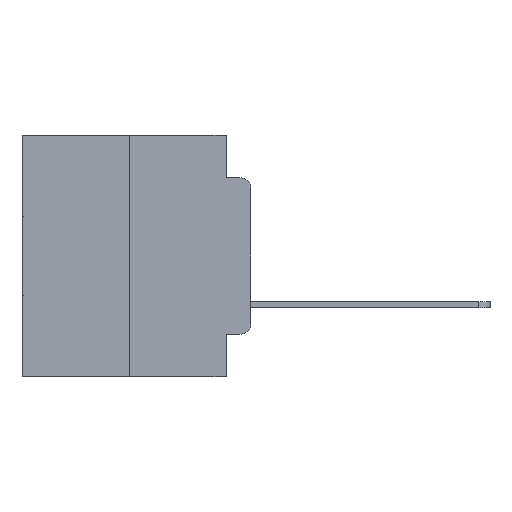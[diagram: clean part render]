
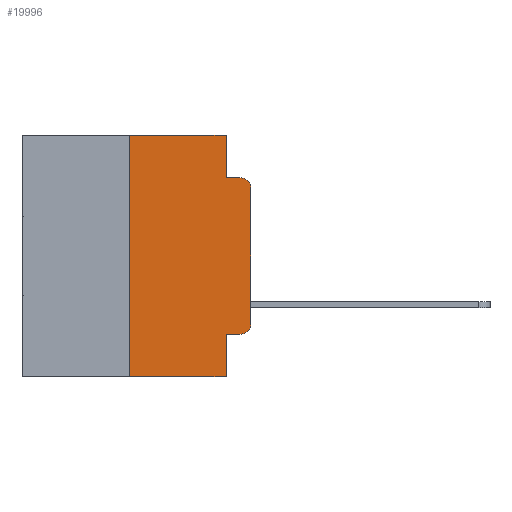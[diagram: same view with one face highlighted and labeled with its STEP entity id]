
A CAD part, left-side view. The second image highlights one B-rep face of the part: STEP entity #19996.
In plain terms, the highlighted planar face has unit normal (-1, 0, 0).
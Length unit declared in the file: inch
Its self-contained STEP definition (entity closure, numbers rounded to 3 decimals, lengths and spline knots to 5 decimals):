
#193 = LINE ( 'NONE', #30476, #29008 ) ;
#1027 = CARTESIAN_POINT ( 'NONE',  ( 0., 0.02, -0.3915 ) ) ;
#1249 = AXIS2_PLACEMENT_3D ( 'NONE', #13235, #3871, #13334 ) ;
#1542 = CARTESIAN_POINT ( 'NONE',  ( 0., 0.25, -0.5 ) ) ;
#2367 = CARTESIAN_POINT ( 'NONE',  ( 0., 0.051, 0. ) ) ;
#2440 = EDGE_CURVE ( 'NONE', #16428, #4167, #28844, .T. ) ;
#2638 = ORIENTED_EDGE ( 'NONE', *, *, #27464, .F. ) ;
#2759 = EDGE_CURVE ( 'NONE', #3921, #19674, #23719, .T. ) ;
#3078 = ORIENTED_EDGE ( 'NONE', *, *, #21939, .T. ) ;
#3146 = VERTEX_POINT ( 'NONE', #27027 ) ;
#3871 = DIRECTION ( 'NONE',  ( -1., 0., 0. ) ) ;
#3921 = VERTEX_POINT ( 'NONE', #7531 ) ;
#4154 = VECTOR ( 'NONE', #22810, 39.37008 ) ;
#4167 = VERTEX_POINT ( 'NONE', #11001 ) ;
#4545 = AXIS2_PLACEMENT_3D ( 'NONE', #23307, #21207, #23595 ) ;
#5847 = EDGE_CURVE ( 'NONE', #24792, #19674, #14619, .T. ) ;
#6753 = ORIENTED_EDGE ( 'NONE', *, *, #13434, .T. ) ;
#7026 = PLANE ( 'NONE',  #4545 ) ;
#7531 = CARTESIAN_POINT ( 'NONE',  ( 0., 0.051, -0.0885 ) ) ;
#7858 = CARTESIAN_POINT ( 'NONE',  ( 0., 0., -0.1085 ) ) ;
#9597 = VECTOR ( 'NONE', #17127, 39.37008 ) ;
#10564 = CIRCLE ( 'NONE', #28488, 0.02 ) ;
#10743 = VERTEX_POINT ( 'NONE', #24425 ) ;
#11001 = CARTESIAN_POINT ( 'NONE',  ( 0., 0.051, -0.5 ) ) ;
#11068 = VERTEX_POINT ( 'NONE', #22005 ) ;
#11670 = DIRECTION ( 'NONE',  ( 0., 0., 1. ) ) ;
#12167 = ORIENTED_EDGE ( 'NONE', *, *, #18716, .F. ) ;
#12281 = EDGE_CURVE ( 'NONE', #11068, #24792, #22073, .T. ) ;
#12638 = LINE ( 'NONE', #24108, #28834 ) ;
#12722 = DIRECTION ( 'NONE',  ( -1., 0., 0. ) ) ;
#13136 = DIRECTION ( 'NONE',  ( 0., -1., 0. ) ) ;
#13235 = CARTESIAN_POINT ( 'NONE',  ( 0., 0.02, -0.1085 ) ) ;
#13334 = DIRECTION ( 'NONE',  ( 0., 0., -1. ) ) ;
#13434 = EDGE_CURVE ( 'NONE', #10743, #11068, #10564, .T. ) ;
#14483 = CARTESIAN_POINT ( 'NONE',  ( 0., 0.25, 0. ) ) ;
#14619 = CIRCLE ( 'NONE', #1249, 0.02 ) ;
#14818 = LINE ( 'NONE', #27575, #23702 ) ;
#15040 = DIRECTION ( 'NONE',  ( 0., -1., 0. ) ) ;
#15348 = EDGE_CURVE ( 'NONE', #27778, #16072, #193, .T. ) ;
#15580 = ORIENTED_EDGE ( 'NONE', *, *, #19689, .T. ) ;
#15909 = LINE ( 'NONE', #24748, #21782 ) ;
#15996 = ORIENTED_EDGE ( 'NONE', *, *, #12281, .T. ) ;
#16072 = VERTEX_POINT ( 'NONE', #14483 ) ;
#16428 = VERTEX_POINT ( 'NONE', #18383 ) ;
#17127 = DIRECTION ( 'NONE',  ( 0., 0., -1. ) ) ;
#18071 = FACE_OUTER_BOUND ( 'NONE', #28025, .T. ) ;
#18383 = CARTESIAN_POINT ( 'NONE',  ( 0., 0.051, -0.4115 ) ) ;
#18716 = EDGE_CURVE ( 'NONE', #16072, #3146, #12638, .T. ) ;
#19674 = VERTEX_POINT ( 'NONE', #24135 ) ;
#19689 = EDGE_CURVE ( 'NONE', #16428, #10743, #15909, .T. ) ;
#19996 = ADVANCED_FACE ( 'NONE', ( #18071 ), #7026, .F. ) ;
#20050 = CARTESIAN_POINT ( 'NONE',  ( 0., 0., 0. ) ) ;
#21207 = DIRECTION ( 'NONE',  ( 1., 0., 0. ) ) ;
#21218 = ORIENTED_EDGE ( 'NONE', *, *, #2440, .F. ) ;
#21608 = DIRECTION ( 'NONE',  ( 0., -1., 0. ) ) ;
#21782 = VECTOR ( 'NONE', #15040, 39.37008 ) ;
#21939 = EDGE_CURVE ( 'NONE', #27778, #4167, #14818, .T. ) ;
#21992 = DIRECTION ( 'NONE',  ( 0., 0., -1. ) ) ;
#22005 = CARTESIAN_POINT ( 'NONE',  ( 0., 0., -0.3915 ) ) ;
#22073 = LINE ( 'NONE', #20050, #23187 ) ;
#22112 = LINE ( 'NONE', #28864, #9597 ) ;
#22610 = CARTESIAN_POINT ( 'NONE',  ( 0., 0.051, -0.0885 ) ) ;
#22804 = ORIENTED_EDGE ( 'NONE', *, *, #15348, .F. ) ;
#22810 = DIRECTION ( 'NONE',  ( 0., -1., 0. ) ) ;
#23187 = VECTOR ( 'NONE', #27902, 39.37008 ) ;
#23307 = CARTESIAN_POINT ( 'NONE',  ( 0., 0.473, 0. ) ) ;
#23595 = DIRECTION ( 'NONE',  ( 0., 0., -1. ) ) ;
#23702 = VECTOR ( 'NONE', #13136, 39.37008 ) ;
#23719 = LINE ( 'NONE', #22610, #4154 ) ;
#24108 = CARTESIAN_POINT ( 'NONE',  ( 0., 0.473, 0. ) ) ;
#24135 = CARTESIAN_POINT ( 'NONE',  ( 0., 0.02, -0.0885 ) ) ;
#24425 = CARTESIAN_POINT ( 'NONE',  ( 0., 0.02, -0.4115 ) ) ;
#24659 = ORIENTED_EDGE ( 'NONE', *, *, #5847, .T. ) ;
#24748 = CARTESIAN_POINT ( 'NONE',  ( 0., 0.051, -0.4115 ) ) ;
#24792 = VERTEX_POINT ( 'NONE', #7858 ) ;
#25552 = ORIENTED_EDGE ( 'NONE', *, *, #2759, .F. ) ;
#27027 = CARTESIAN_POINT ( 'NONE',  ( 0., 0.051, 0. ) ) ;
#27412 = VECTOR ( 'NONE', #30502, 39.37008 ) ;
#27464 = EDGE_CURVE ( 'NONE', #3146, #3921, #22112, .T. ) ;
#27575 = CARTESIAN_POINT ( 'NONE',  ( 0., 0.473, -0.5 ) ) ;
#27778 = VERTEX_POINT ( 'NONE', #1542 ) ;
#27902 = DIRECTION ( 'NONE',  ( 0., 0., 1. ) ) ;
#28025 = EDGE_LOOP ( 'NONE', ( #15996, #24659, #25552, #2638, #12167, #22804, #3078, #21218, #15580, #6753 ) ) ;
#28488 = AXIS2_PLACEMENT_3D ( 'NONE', #1027, #12722, #21992 ) ;
#28834 = VECTOR ( 'NONE', #21608, 39.37008 ) ;
#28844 = LINE ( 'NONE', #2367, #27412 ) ;
#28864 = CARTESIAN_POINT ( 'NONE',  ( 0., 0.051, 0. ) ) ;
#29008 = VECTOR ( 'NONE', #11670, 39.37008 ) ;
#30476 = CARTESIAN_POINT ( 'NONE',  ( 0., 0.25, 0. ) ) ;
#30502 = DIRECTION ( 'NONE',  ( 0., 0., -1. ) ) ;
